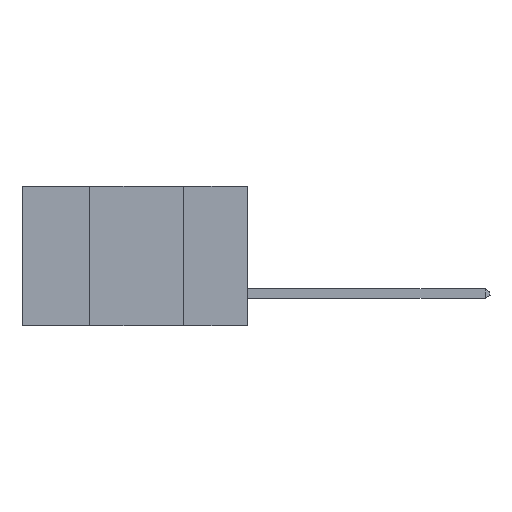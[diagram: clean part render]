
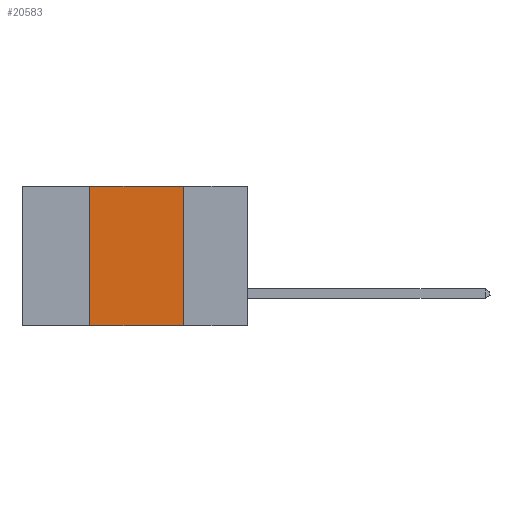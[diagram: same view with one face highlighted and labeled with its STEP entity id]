
A CAD part, left-side view. The second image highlights one B-rep face of the part: STEP entity #20583.
In plain terms, the highlighted planar face has unit normal (-1, 0, 0).
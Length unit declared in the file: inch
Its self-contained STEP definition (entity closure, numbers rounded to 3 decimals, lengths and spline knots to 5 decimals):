
#101 = LINE ( 'NONE', #3551, #20063 ) ;
#370 = AXIS2_PLACEMENT_3D ( 'NONE', #9321, #4576, #17447 ) ;
#515 = FACE_OUTER_BOUND ( 'NONE', #10829, .T. ) ;
#1094 = DIRECTION ( 'NONE',  ( 0., 0., -1. ) ) ;
#1155 = LINE ( 'NONE', #1190, #9202 ) ;
#1190 = CARTESIAN_POINT ( 'NONE',  ( 0., 0.6, 0. ) ) ;
#1838 = EDGE_CURVE ( 'NONE', #16907, #15993, #1155, .T. ) ;
#1918 = DIRECTION ( 'NONE',  ( 0., -1., 0. ) ) ;
#3551 = CARTESIAN_POINT ( 'NONE',  ( 0., 0.42, 0. ) ) ;
#3601 = ORIENTED_EDGE ( 'NONE', *, *, #6580, .F. ) ;
#3619 = CARTESIAN_POINT ( 'NONE',  ( 0., 0.17, 0. ) ) ;
#4157 = CARTESIAN_POINT ( 'NONE',  ( 0., 0.17, 0. ) ) ;
#4576 = DIRECTION ( 'NONE',  ( 1., 0., 0. ) ) ;
#5670 = VECTOR ( 'NONE', #1918, 39.37008 ) ;
#5722 = VERTEX_POINT ( 'NONE', #15067 ) ;
#6578 = ORIENTED_EDGE ( 'NONE', *, *, #13539, .T. ) ;
#6580 = EDGE_CURVE ( 'NONE', #15993, #6881, #8389, .T. ) ;
#6740 = CARTESIAN_POINT ( 'NONE',  ( 0., 0.6, -0.37 ) ) ;
#6881 = VERTEX_POINT ( 'NONE', #11336 ) ;
#7580 = DIRECTION ( 'NONE',  ( 0., -1., 0. ) ) ;
#8154 = ORIENTED_EDGE ( 'NONE', *, *, #11058, .F. ) ;
#8389 = LINE ( 'NONE', #4157, #18741 ) ;
#9202 = VECTOR ( 'NONE', #7580, 39.37008 ) ;
#9321 = CARTESIAN_POINT ( 'NONE',  ( 0., 0.6, 0. ) ) ;
#10231 = DIRECTION ( 'NONE',  ( 0., 0., 1. ) ) ;
#10827 = CARTESIAN_POINT ( 'NONE',  ( 0., 0.42, 0. ) ) ;
#10829 = EDGE_LOOP ( 'NONE', ( #3601, #20801, #8154, #6578 ) ) ;
#11058 = EDGE_CURVE ( 'NONE', #5722, #16907, #101, .T. ) ;
#11336 = CARTESIAN_POINT ( 'NONE',  ( 0., 0.17, -0.37 ) ) ;
#13539 = EDGE_CURVE ( 'NONE', #5722, #6881, #17038, .T. ) ;
#15067 = CARTESIAN_POINT ( 'NONE',  ( 0., 0.42, -0.37 ) ) ;
#15993 = VERTEX_POINT ( 'NONE', #3619 ) ;
#16907 = VERTEX_POINT ( 'NONE', #10827 ) ;
#17038 = LINE ( 'NONE', #6740, #5670 ) ;
#17447 = DIRECTION ( 'NONE',  ( 0., 0., -1. ) ) ;
#18741 = VECTOR ( 'NONE', #1094, 39.37008 ) ;
#18925 = PLANE ( 'NONE',  #370 ) ;
#20063 = VECTOR ( 'NONE', #10231, 39.37008 ) ;
#20583 = ADVANCED_FACE ( 'NONE', ( #515 ), #18925, .F. ) ;
#20801 = ORIENTED_EDGE ( 'NONE', *, *, #1838, .F. ) ;
